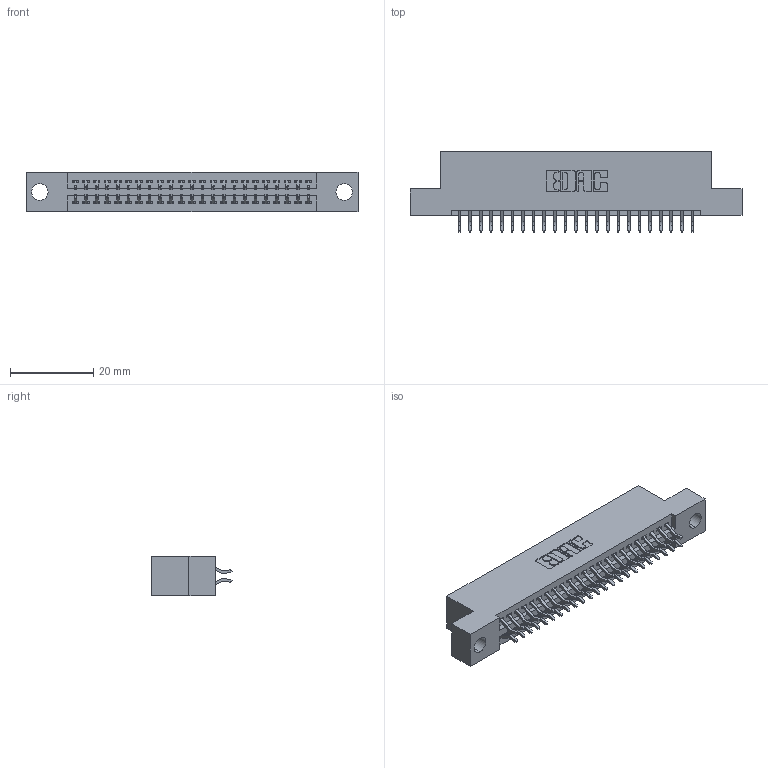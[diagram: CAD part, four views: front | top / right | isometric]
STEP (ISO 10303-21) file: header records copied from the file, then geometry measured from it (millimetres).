
FILE_DESCRIPTION (( 'STEP AP203' ), '1' );
FILE_NAME ('395-046-556-204.STEP', '2021-06-16T23:10:31', ( '' ), ( '' ), 'SwSTEP 2.0', 'SolidWorks 2020', '' );
FILE_SCHEMA (( 'CONFIG_CONTROL_DESIGN' ));
Length unit declared in the file: inch
Products named in the file (3): 345 Part_Flush Mounting Lugs - 0.156 Dia-TI; 345-292-001_556 Tail; 395-046-556-204
Assembly tree (47 placements, depth 2):
  395-046-556-204
    345 Part_Flush Mounting Lugs - 0.156 Dia-TI
    345-292-001_556 Tail  x46
Bounding box: 79.63 x 19.24 x 9.4 mm (x, y, z)
Volume: 7451.1 mm3; surface area: 10457.3 mm2
Topology: 47 solids, 47 shells, 2716 faces, 8059 edges, 5310 vertices
Faces by surface type: plane 1796, cylinder 920
Entity records: 21243 total; most frequent: CARTESIAN_POINT 3598, ORIENTED_EDGE 3518, DIRECTION 3183, EDGE_CURVE 1759, VECTOR 1527, LINE 1527, VERTEX_POINT 1170, AXIS2_PLACEMENT_3D 828
